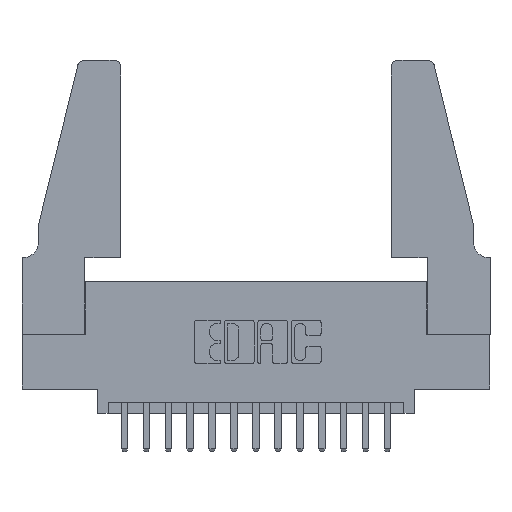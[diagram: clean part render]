
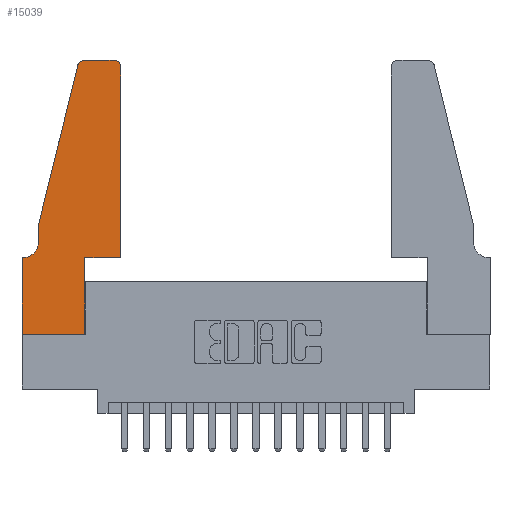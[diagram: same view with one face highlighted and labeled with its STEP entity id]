
A CAD part, top view. The second image highlights one B-rep face of the part: STEP entity #15039.
In plain terms, the highlighted planar face has unit normal (0, 0, 1).
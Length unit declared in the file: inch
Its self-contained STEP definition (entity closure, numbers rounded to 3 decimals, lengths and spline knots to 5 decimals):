
#337 = AXIS2_PLACEMENT_3D ( 'NONE', #3475, #12383, #13709 ) ;
#400 = DIRECTION ( 'NONE',  ( 0., 1., 0. ) ) ;
#550 = EDGE_CURVE ( 'NONE', #9224, #5100, #5539, .T. ) ;
#684 = CARTESIAN_POINT ( 'NONE',  ( 0.4505, 1.22, 0.37 ) ) ;
#789 = LINE ( 'NONE', #16203, #15974 ) ;
#818 = CARTESIAN_POINT ( 'NONE',  ( 0.0755, 0.5, 0.37 ) ) ;
#978 = DIRECTION ( 'NONE',  ( -1., 0., 0. ) ) ;
#1005 = DIRECTION ( 'NONE',  ( -1., 0., 0. ) ) ;
#2110 = CARTESIAN_POINT ( 'NONE',  ( 0., 0., 0.37 ) ) ;
#2172 = CARTESIAN_POINT ( 'NONE',  ( 0.0755, 0.42, 0.37 ) ) ;
#2897 = CARTESIAN_POINT ( 'NONE',  ( 0.4505, 0.35, 0.37 ) ) ;
#3314 = VERTEX_POINT ( 'NONE', #2897 ) ;
#3475 = CARTESIAN_POINT ( 'NONE',  ( 0.4205, 1.22, 0.37 ) ) ;
#3559 = CARTESIAN_POINT ( 'NONE',  ( 0.2865, 0., 0.37 ) ) ;
#3734 = DIRECTION ( 'NONE',  ( 0., 0., 1. ) ) ;
#3856 = CARTESIAN_POINT ( 'NONE',  ( 0.284, 1.22, 0.37 ) ) ;
#3894 = ORIENTED_EDGE ( 'NONE', *, *, #9591, .T. ) ;
#4037 = LINE ( 'NONE', #9743, #12388 ) ;
#4161 = EDGE_CURVE ( 'NONE', #5634, #5397, #5821, .T. ) ;
#4437 = DIRECTION ( 'NONE',  ( 1., 0., 0. ) ) ;
#4447 = DIRECTION ( 'NONE',  ( 1., 0., 0. ) ) ;
#4666 = CIRCLE ( 'NONE', #9822, 0.07 ) ;
#4691 = ORIENTED_EDGE ( 'NONE', *, *, #9112, .T. ) ;
#4915 = LINE ( 'NONE', #11408, #5902 ) ;
#4970 = VECTOR ( 'NONE', #13672, 39.37008 ) ;
#5015 = DIRECTION ( 'NONE',  ( 1., 0., 0. ) ) ;
#5100 = VERTEX_POINT ( 'NONE', #12044 ) ;
#5162 = EDGE_CURVE ( 'NONE', #11473, #9805, #4666, .T. ) ;
#5198 = VECTOR ( 'NONE', #1005, 39.37008 ) ;
#5361 = LINE ( 'NONE', #12918, #13550 ) ;
#5397 = VERTEX_POINT ( 'NONE', #13002 ) ;
#5539 = LINE ( 'NONE', #818, #9736 ) ;
#5614 = VERTEX_POINT ( 'NONE', #10770 ) ;
#5634 = VERTEX_POINT ( 'NONE', #3559 ) ;
#5821 = LINE ( 'NONE', #14814, #13827 ) ;
#5875 = CARTESIAN_POINT ( 'NONE',  ( 0.284, 1.25, 0.37 ) ) ;
#5902 = VECTOR ( 'NONE', #978, 39.37008 ) ;
#5975 = DIRECTION ( 'NONE',  ( 0., 0., -1. ) ) ;
#6231 = EDGE_CURVE ( 'NONE', #5397, #3314, #4037, .T. ) ;
#6573 = CARTESIAN_POINT ( 'NONE',  ( 0.0755, 0.5, 0.37 ) ) ;
#6645 = EDGE_CURVE ( 'NONE', #11399, #14179, #789, .T. ) ;
#6790 = ORIENTED_EDGE ( 'NONE', *, *, #14211, .T. ) ;
#7046 = EDGE_CURVE ( 'NONE', #5614, #15878, #8188, .T. ) ;
#7670 = EDGE_CURVE ( 'NONE', #14179, #5634, #14945, .T. ) ;
#7744 = DIRECTION ( 'NONE',  ( 0., -1., 0. ) ) ;
#7804 = VERTEX_POINT ( 'NONE', #684 ) ;
#8026 = ORIENTED_EDGE ( 'NONE', *, *, #7670, .T. ) ;
#8090 = EDGE_LOOP ( 'NONE', ( #10840, #4691, #12615, #6790, #9376, #12696, #14199, #8026, #16186, #13106, #8916, #3894 ) ) ;
#8109 = FACE_OUTER_BOUND ( 'NONE', #8090, .T. ) ;
#8112 = EDGE_CURVE ( 'NONE', #3314, #7804, #5361, .T. ) ;
#8188 = LINE ( 'NONE', #13640, #5198 ) ;
#8340 = CIRCLE ( 'NONE', #12740, 0.03 ) ;
#8418 = AXIS2_PLACEMENT_3D ( 'NONE', #9572, #13417, #4437 ) ;
#8563 = DIRECTION ( 'NONE',  ( 0., -1., 0. ) ) ;
#8737 = VECTOR ( 'NONE', #7744, 39.37008 ) ;
#8916 = ORIENTED_EDGE ( 'NONE', *, *, #8112, .T. ) ;
#9112 = EDGE_CURVE ( 'NONE', #15878, #9224, #8340, .T. ) ;
#9224 = VERTEX_POINT ( 'NONE', #15500 ) ;
#9376 = ORIENTED_EDGE ( 'NONE', *, *, #5162, .T. ) ;
#9551 = LINE ( 'NONE', #6573, #8737 ) ;
#9572 = CARTESIAN_POINT ( 'NONE',  ( 0., 0.35, 0.37 ) ) ;
#9591 = EDGE_CURVE ( 'NONE', #7804, #5614, #9928, .T. ) ;
#9736 = VECTOR ( 'NONE', #15055, 39.37008 ) ;
#9743 = CARTESIAN_POINT ( 'NONE',  ( 0.4505, 0.35, 0.37 ) ) ;
#9805 = VERTEX_POINT ( 'NONE', #10445 ) ;
#9822 = AXIS2_PLACEMENT_3D ( 'NONE', #13638, #5975, #14904 ) ;
#9928 = CIRCLE ( 'NONE', #337, 0.03 ) ;
#10085 = EDGE_CURVE ( 'NONE', #9805, #11399, #4915, .T. ) ;
#10445 = CARTESIAN_POINT ( 'NONE',  ( 0.0055, 0.35, 0.37 ) ) ;
#10770 = CARTESIAN_POINT ( 'NONE',  ( 0.4205, 1.25, 0.37 ) ) ;
#10840 = ORIENTED_EDGE ( 'NONE', *, *, #7046, .T. ) ;
#10868 = DIRECTION ( 'NONE',  ( 0., 1., 0. ) ) ;
#11322 = CARTESIAN_POINT ( 'NONE',  ( 0., 0.35, 0.37 ) ) ;
#11399 = VERTEX_POINT ( 'NONE', #11322 ) ;
#11408 = CARTESIAN_POINT ( 'NONE',  ( 0.0755, 0.35, 0.37 ) ) ;
#11473 = VERTEX_POINT ( 'NONE', #2172 ) ;
#11480 = CARTESIAN_POINT ( 'NONE',  ( 0., 0., 0.37 ) ) ;
#12044 = CARTESIAN_POINT ( 'NONE',  ( 0.0755, 0.5, 0.37 ) ) ;
#12383 = DIRECTION ( 'NONE',  ( 0., 0., 1. ) ) ;
#12388 = VECTOR ( 'NONE', #4447, 39.37008 ) ;
#12615 = ORIENTED_EDGE ( 'NONE', *, *, #550, .T. ) ;
#12696 = ORIENTED_EDGE ( 'NONE', *, *, #10085, .T. ) ;
#12740 = AXIS2_PLACEMENT_3D ( 'NONE', #3856, #3734, #5015 ) ;
#12918 = CARTESIAN_POINT ( 'NONE',  ( 0.4505, 0.35, 0.37 ) ) ;
#13002 = CARTESIAN_POINT ( 'NONE',  ( 0.2865, 0.35, 0.37 ) ) ;
#13106 = ORIENTED_EDGE ( 'NONE', *, *, #6231, .T. ) ;
#13417 = DIRECTION ( 'NONE',  ( 0., 0., 1. ) ) ;
#13550 = VECTOR ( 'NONE', #400, 39.37008 ) ;
#13638 = CARTESIAN_POINT ( 'NONE',  ( 0.0055, 0.42, 0.37 ) ) ;
#13640 = CARTESIAN_POINT ( 'NONE',  ( 0.2605, 1.25, 0.37 ) ) ;
#13672 = DIRECTION ( 'NONE',  ( 1., 0., 0. ) ) ;
#13709 = DIRECTION ( 'NONE',  ( 1., 0., 0. ) ) ;
#13827 = VECTOR ( 'NONE', #10868, 39.37008 ) ;
#14179 = VERTEX_POINT ( 'NONE', #11480 ) ;
#14199 = ORIENTED_EDGE ( 'NONE', *, *, #6645, .T. ) ;
#14211 = EDGE_CURVE ( 'NONE', #5100, #11473, #9551, .T. ) ;
#14688 = PLANE ( 'NONE',  #8418 ) ;
#14814 = CARTESIAN_POINT ( 'NONE',  ( 0.2865, 0.35, 0.37 ) ) ;
#14904 = DIRECTION ( 'NONE',  ( -1., 0., 0. ) ) ;
#14945 = LINE ( 'NONE', #2110, #4970 ) ;
#15039 = ADVANCED_FACE ( 'NONE', ( #8109 ), #14688, .T. ) ;
#15055 = DIRECTION ( 'NONE',  ( -0.239, -0.971, 0. ) ) ;
#15500 = CARTESIAN_POINT ( 'NONE',  ( 0.25487, 1.22718, 0.37 ) ) ;
#15878 = VERTEX_POINT ( 'NONE', #5875 ) ;
#15974 = VECTOR ( 'NONE', #8563, 39.37008 ) ;
#16186 = ORIENTED_EDGE ( 'NONE', *, *, #4161, .T. ) ;
#16203 = CARTESIAN_POINT ( 'NONE',  ( 0., 0., 0.37 ) ) ;
